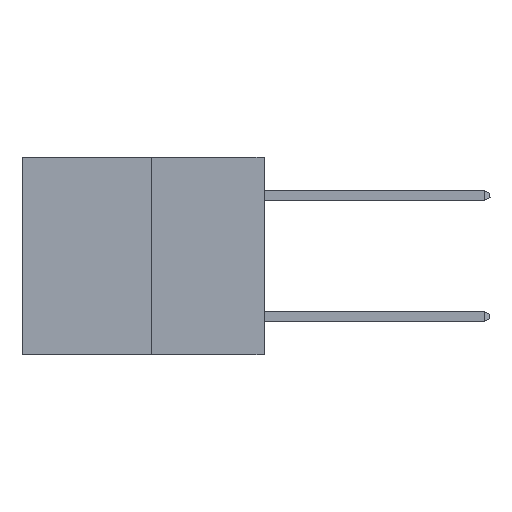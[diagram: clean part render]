
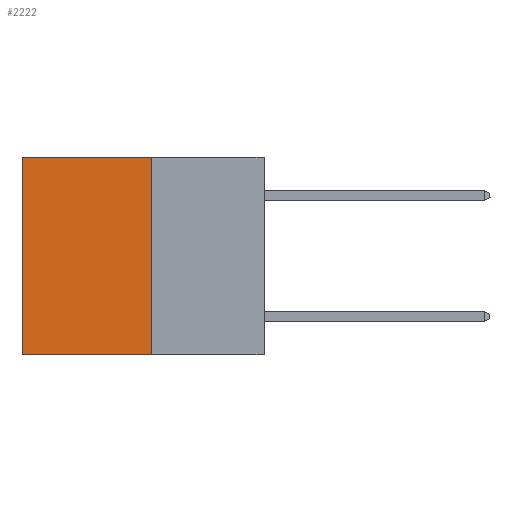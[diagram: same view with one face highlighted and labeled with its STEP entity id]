
A CAD part, left-side view. The second image highlights one B-rep face of the part: STEP entity #2222.
In plain terms, the highlighted planar face has unit normal (-1, 0, 0).
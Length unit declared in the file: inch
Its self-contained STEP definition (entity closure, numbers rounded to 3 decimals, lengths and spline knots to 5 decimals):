
#98 = CARTESIAN_POINT ( 'NONE',  ( 0.3165, 0.28, -0.49 ) ) ;
#1194 = ORIENTED_EDGE ( 'NONE', *, *, #17116, .F. ) ;
#1841 = ORIENTED_EDGE ( 'NONE', *, *, #5777, .T. ) ;
#1861 = DIRECTION ( 'NONE',  ( 0., 1., 0. ) ) ;
#2222 = ADVANCED_FACE ( 'NONE', ( #3032 ), #2624, .F. ) ;
#2624 = PLANE ( 'NONE',  #10160 ) ;
#2851 = VERTEX_POINT ( 'NONE', #6429 ) ;
#3032 = FACE_OUTER_BOUND ( 'NONE', #7270, .T. ) ;
#3735 = LINE ( 'NONE', #23169, #5540 ) ;
#4692 = VERTEX_POINT ( 'NONE', #8894 ) ;
#4882 = VERTEX_POINT ( 'NONE', #20124 ) ;
#5540 = VECTOR ( 'NONE', #1861, 39.37008 ) ;
#5635 = CARTESIAN_POINT ( 'NONE',  ( 0.3165, 0.28, 0. ) ) ;
#5777 = EDGE_CURVE ( 'NONE', #2851, #4692, #9748, .T. ) ;
#6162 = VERTEX_POINT ( 'NONE', #9012 ) ;
#6429 = CARTESIAN_POINT ( 'NONE',  ( 0.3165, 0.6, 0. ) ) ;
#7270 = EDGE_LOOP ( 'NONE', ( #1841, #17093, #1194, #16541 ) ) ;
#8502 = VECTOR ( 'NONE', #21938, 39.37008 ) ;
#8894 = CARTESIAN_POINT ( 'NONE',  ( 0.3165, 0.6, -0.49 ) ) ;
#9012 = CARTESIAN_POINT ( 'NONE',  ( 0.3165, 0.28, -0.49 ) ) ;
#9732 = DIRECTION ( 'NONE',  ( 0., 0., -1. ) ) ;
#9748 = LINE ( 'NONE', #28694, #27631 ) ;
#10160 = AXIS2_PLACEMENT_3D ( 'NONE', #12115, #14596, #28323 ) ;
#12115 = CARTESIAN_POINT ( 'NONE',  ( 0.3165, 0.28, -0.49 ) ) ;
#14527 = LINE ( 'NONE', #98, #27353 ) ;
#14596 = DIRECTION ( 'NONE',  ( 1., 0., 0. ) ) ;
#15486 = DIRECTION ( 'NONE',  ( 0., 0., -1. ) ) ;
#16541 = ORIENTED_EDGE ( 'NONE', *, *, #19152, .T. ) ;
#17093 = ORIENTED_EDGE ( 'NONE', *, *, #20484, .F. ) ;
#17116 = EDGE_CURVE ( 'NONE', #4882, #6162, #14527, .T. ) ;
#19091 = LINE ( 'NONE', #5635, #8502 ) ;
#19152 = EDGE_CURVE ( 'NONE', #4882, #2851, #19091, .T. ) ;
#20124 = CARTESIAN_POINT ( 'NONE',  ( 0.3165, 0.28, 0. ) ) ;
#20484 = EDGE_CURVE ( 'NONE', #6162, #4692, #3735, .T. ) ;
#21938 = DIRECTION ( 'NONE',  ( 0., 1., 0. ) ) ;
#23169 = CARTESIAN_POINT ( 'NONE',  ( 0.3165, 0.28, -0.49 ) ) ;
#27353 = VECTOR ( 'NONE', #9732, 39.37008 ) ;
#27631 = VECTOR ( 'NONE', #15486, 39.37008 ) ;
#28323 = DIRECTION ( 'NONE',  ( 0., 0., -1. ) ) ;
#28694 = CARTESIAN_POINT ( 'NONE',  ( 0.3165, 0.6, -0.49 ) ) ;
